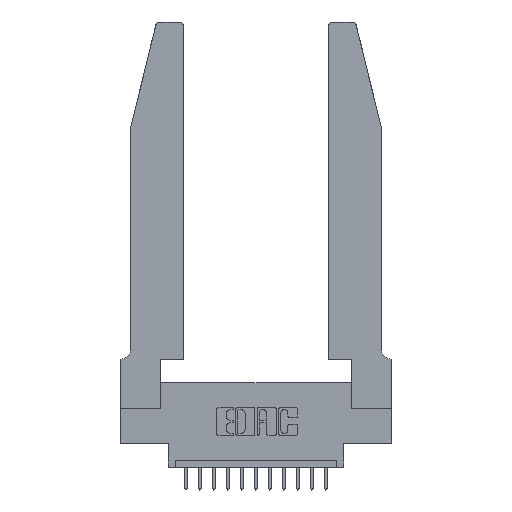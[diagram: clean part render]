
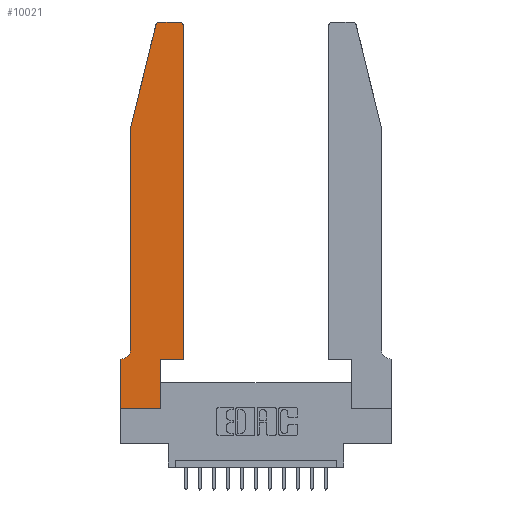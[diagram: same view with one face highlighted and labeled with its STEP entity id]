
A CAD part, top view. The second image highlights one B-rep face of the part: STEP entity #10021.
In plain terms, the highlighted planar face has unit normal (0, 0, 1).
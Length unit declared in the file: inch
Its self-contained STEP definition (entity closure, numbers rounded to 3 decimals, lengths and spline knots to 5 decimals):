
#4 = VECTOR ( 'NONE', #13313, 39.37008 ) ;
#146 = EDGE_CURVE ( 'NONE', #6314, #5536, #16015, .T. ) ;
#206 = LINE ( 'NONE', #14562, #4 ) ;
#311 = CARTESIAN_POINT ( 'NONE',  ( 0.284, 2.75, 0.37 ) ) ;
#601 = VECTOR ( 'NONE', #9963, 39.37008 ) ;
#684 = VECTOR ( 'NONE', #4437, 39.37008 ) ;
#1062 = DIRECTION ( 'NONE',  ( 0., 0., 1. ) ) ;
#1247 = ORIENTED_EDGE ( 'NONE', *, *, #3881, .T. ) ;
#1416 = PLANE ( 'NONE',  #15054 ) ;
#1460 = EDGE_CURVE ( 'NONE', #2772, #6314, #5578, .T. ) ;
#1639 = LINE ( 'NONE', #12577, #2314 ) ;
#1662 = VERTEX_POINT ( 'NONE', #13258 ) ;
#1678 = VERTEX_POINT ( 'NONE', #9320 ) ;
#1722 = CARTESIAN_POINT ( 'NONE',  ( 0., 0., 0.37 ) ) ;
#1777 = ORIENTED_EDGE ( 'NONE', *, *, #4565, .T. ) ;
#1796 = VERTEX_POINT ( 'NONE', #9661 ) ;
#2314 = VECTOR ( 'NONE', #5983, 39.37008 ) ;
#2772 = VERTEX_POINT ( 'NONE', #5819 ) ;
#2825 = VERTEX_POINT ( 'NONE', #11401 ) ;
#2876 = ORIENTED_EDGE ( 'NONE', *, *, #1460, .T. ) ;
#2918 = CARTESIAN_POINT ( 'NONE',  ( 0., 0.35, 0.37 ) ) ;
#3070 = CARTESIAN_POINT ( 'NONE',  ( 0.4505, 0.35, 0.37 ) ) ;
#3202 = ORIENTED_EDGE ( 'NONE', *, *, #14744, .T. ) ;
#3386 = CIRCLE ( 'NONE', #9881, 0.03 ) ;
#3881 = EDGE_CURVE ( 'NONE', #1678, #1662, #16411, .T. ) ;
#4437 = DIRECTION ( 'NONE',  ( 0., 1., 0. ) ) ;
#4556 = VERTEX_POINT ( 'NONE', #6773 ) ;
#4565 = EDGE_CURVE ( 'NONE', #1796, #15322, #10707, .T. ) ;
#5399 = DIRECTION ( 'NONE',  ( 0., 0., 1. ) ) ;
#5416 = CARTESIAN_POINT ( 'NONE',  ( 0., 0., 0.37 ) ) ;
#5425 = ORIENTED_EDGE ( 'NONE', *, *, #10987, .T. ) ;
#5536 = VERTEX_POINT ( 'NONE', #12347 ) ;
#5578 = LINE ( 'NONE', #5734, #11460 ) ;
#5625 = EDGE_CURVE ( 'NONE', #2825, #8994, #12362, .T. ) ;
#5734 = CARTESIAN_POINT ( 'NONE',  ( 0.4505, 0.35, 0.37 ) ) ;
#5819 = CARTESIAN_POINT ( 'NONE',  ( 0.2865, 0.35, 0.37 ) ) ;
#5983 = DIRECTION ( 'NONE',  ( 0., 1., 0. ) ) ;
#6145 = CARTESIAN_POINT ( 'NONE',  ( 0.4205, 2.72, 0.37 ) ) ;
#6314 = VERTEX_POINT ( 'NONE', #3070 ) ;
#6342 = EDGE_CURVE ( 'NONE', #8994, #1678, #8161, .T. ) ;
#6461 = AXIS2_PLACEMENT_3D ( 'NONE', #17180, #6563, #15840 ) ;
#6563 = DIRECTION ( 'NONE',  ( 0., 0., -1. ) ) ;
#6674 = DIRECTION ( 'NONE',  ( 0., -1., 0. ) ) ;
#6741 = ORIENTED_EDGE ( 'NONE', *, *, #146, .T. ) ;
#6773 = CARTESIAN_POINT ( 'NONE',  ( 0.4205, 2.75, 0.37 ) ) ;
#7485 = DIRECTION ( 'NONE',  ( 1., 0., 0. ) ) ;
#7509 = DIRECTION ( 'NONE',  ( -0.239, -0.971, 0. ) ) ;
#7903 = EDGE_CURVE ( 'NONE', #12035, #1796, #14617, .T. ) ;
#8161 = LINE ( 'NONE', #10081, #601 ) ;
#8217 = DIRECTION ( 'NONE',  ( 1., 0., 0. ) ) ;
#8349 = CARTESIAN_POINT ( 'NONE',  ( 0.4505, 0.35, 0.37 ) ) ;
#8909 = VERTEX_POINT ( 'NONE', #311 ) ;
#8964 = VECTOR ( 'NONE', #15660, 39.37008 ) ;
#8994 = VERTEX_POINT ( 'NONE', #16039 ) ;
#9246 = EDGE_CURVE ( 'NONE', #5536, #4556, #16450, .T. ) ;
#9320 = CARTESIAN_POINT ( 'NONE',  ( 0.0755, 0.42, 0.37 ) ) ;
#9599 = ORIENTED_EDGE ( 'NONE', *, *, #9246, .T. ) ;
#9661 = CARTESIAN_POINT ( 'NONE',  ( 0., 0., 0.37 ) ) ;
#9881 = AXIS2_PLACEMENT_3D ( 'NONE', #10486, #1062, #10431 ) ;
#9963 = DIRECTION ( 'NONE',  ( 0., -1., 0. ) ) ;
#10021 = ADVANCED_FACE ( 'NONE', ( #10527 ), #1416, .T. ) ;
#10081 = CARTESIAN_POINT ( 'NONE',  ( 0.0755, 2., 0.37 ) ) ;
#10431 = DIRECTION ( 'NONE',  ( 1., 0., 0. ) ) ;
#10481 = CARTESIAN_POINT ( 'NONE',  ( 0.2865, 0., 0.37 ) ) ;
#10482 = ORIENTED_EDGE ( 'NONE', *, *, #13658, .T. ) ;
#10486 = CARTESIAN_POINT ( 'NONE',  ( 0.284, 2.72, 0.37 ) ) ;
#10527 = FACE_OUTER_BOUND ( 'NONE', #12082, .T. ) ;
#10707 = LINE ( 'NONE', #5416, #16181 ) ;
#10942 = ORIENTED_EDGE ( 'NONE', *, *, #16413, .T. ) ;
#10987 = EDGE_CURVE ( 'NONE', #8909, #2825, #3386, .T. ) ;
#11401 = CARTESIAN_POINT ( 'NONE',  ( 0.25487, 2.72718, 0.37 ) ) ;
#11460 = VECTOR ( 'NONE', #8217, 39.37008 ) ;
#11501 = LINE ( 'NONE', #13120, #8964 ) ;
#11849 = ORIENTED_EDGE ( 'NONE', *, *, #6342, .T. ) ;
#12035 = VERTEX_POINT ( 'NONE', #2918 ) ;
#12082 = EDGE_LOOP ( 'NONE', ( #3202, #5425, #15193, #11849, #1247, #10482, #15414, #1777, #10942, #2876, #6741, #9599 ) ) ;
#12347 = CARTESIAN_POINT ( 'NONE',  ( 0.4505, 2.72, 0.37 ) ) ;
#12362 = LINE ( 'NONE', #16673, #14276 ) ;
#12577 = CARTESIAN_POINT ( 'NONE',  ( 0.2865, 0.35, 0.37 ) ) ;
#12621 = DIRECTION ( 'NONE',  ( 0., 0., 1. ) ) ;
#13120 = CARTESIAN_POINT ( 'NONE',  ( 0.0755, 0.35, 0.37 ) ) ;
#13258 = CARTESIAN_POINT ( 'NONE',  ( 0.0055, 0.35, 0.37 ) ) ;
#13313 = DIRECTION ( 'NONE',  ( -1., 0., 0. ) ) ;
#13362 = CARTESIAN_POINT ( 'NONE',  ( 0., 0.35, 0.37 ) ) ;
#13658 = EDGE_CURVE ( 'NONE', #1662, #12035, #11501, .T. ) ;
#14276 = VECTOR ( 'NONE', #7509, 39.37008 ) ;
#14562 = CARTESIAN_POINT ( 'NONE',  ( 0.2605, 2.75, 0.37 ) ) ;
#14617 = LINE ( 'NONE', #1722, #15033 ) ;
#14744 = EDGE_CURVE ( 'NONE', #4556, #8909, #206, .T. ) ;
#15033 = VECTOR ( 'NONE', #6674, 39.37008 ) ;
#15054 = AXIS2_PLACEMENT_3D ( 'NONE', #13362, #5399, #16196 ) ;
#15193 = ORIENTED_EDGE ( 'NONE', *, *, #5625, .T. ) ;
#15322 = VERTEX_POINT ( 'NONE', #10481 ) ;
#15414 = ORIENTED_EDGE ( 'NONE', *, *, #7903, .T. ) ;
#15660 = DIRECTION ( 'NONE',  ( -1., 0., 0. ) ) ;
#15840 = DIRECTION ( 'NONE',  ( -1., 0., 0. ) ) ;
#16015 = LINE ( 'NONE', #8349, #684 ) ;
#16039 = CARTESIAN_POINT ( 'NONE',  ( 0.0755, 2., 0.37 ) ) ;
#16053 = DIRECTION ( 'NONE',  ( 1., 0., 0. ) ) ;
#16076 = AXIS2_PLACEMENT_3D ( 'NONE', #6145, #12621, #7485 ) ;
#16181 = VECTOR ( 'NONE', #16053, 39.37008 ) ;
#16196 = DIRECTION ( 'NONE',  ( 1., 0., 0. ) ) ;
#16411 = CIRCLE ( 'NONE', #6461, 0.07 ) ;
#16413 = EDGE_CURVE ( 'NONE', #15322, #2772, #1639, .T. ) ;
#16450 = CIRCLE ( 'NONE', #16076, 0.03 ) ;
#16673 = CARTESIAN_POINT ( 'NONE',  ( 0.0755, 2., 0.37 ) ) ;
#17180 = CARTESIAN_POINT ( 'NONE',  ( 0.0055, 0.42, 0.37 ) ) ;
